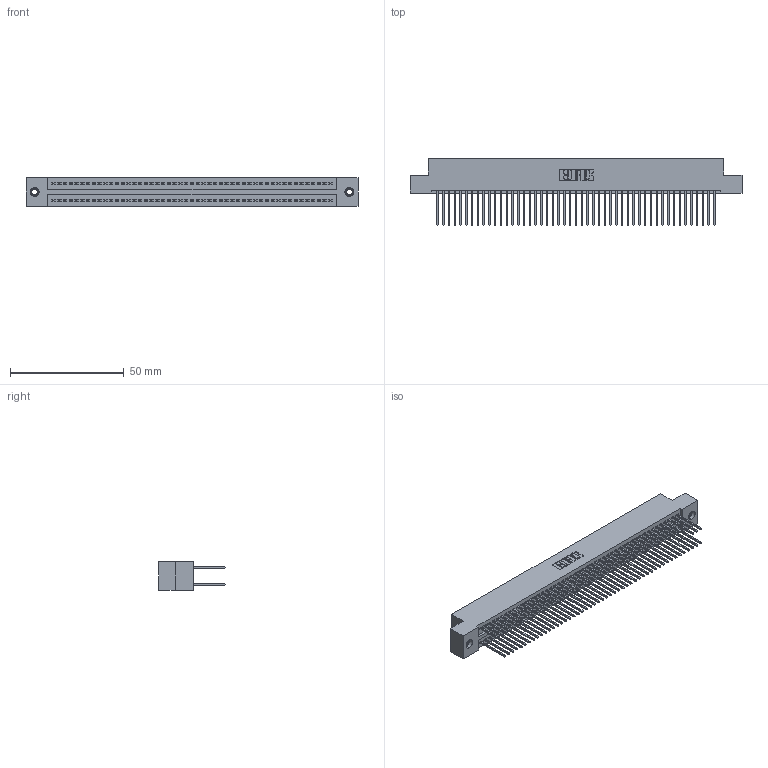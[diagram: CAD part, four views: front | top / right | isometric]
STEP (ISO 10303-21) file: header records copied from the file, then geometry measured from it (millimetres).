
FILE_DESCRIPTION (( 'STEP AP203' ), '1' );
FILE_NAME ('325-098-540-207.STEP', '2020-02-25T06:29:26', ( '' ), ( '' ), 'SwSTEP 2.0', 'SolidWorks 2016', '' );
FILE_SCHEMA (( 'CONFIG_CONTROL_DESIGN' ));
Length unit declared in the file: inch
Products named in the file (4): 325 Part_TI; 325-292-001_325-293-140; 325-098-540-207; 345-250-001_345-250-005-103
Assembly tree (101 placements, depth 2):
  325-098-540-207
    325 Part_TI
    325-292-001_325-293-140  x98
    345-250-001_345-250-005-103  x2
Bounding box: 146.18 x 29.46 x 12.45 mm (x, y, z)
Volume: 19291.8 mm3; surface area: 25310.9 mm2
Topology: 101 solids, 101 shells, 5270 faces, 15637 edges, 10286 vertices
Faces by surface type: plane 3630, cylinder 1624, cone 12, torus 4
Entity records: 31822 total; most frequent: CARTESIAN_POINT 5249, ORIENTED_EDGE 5178, DIRECTION 4503, EDGE_CURVE 2589, LINE 2441, VECTOR 2441, VERTEX_POINT 1720, AXIS2_PLACEMENT_3D 1031
